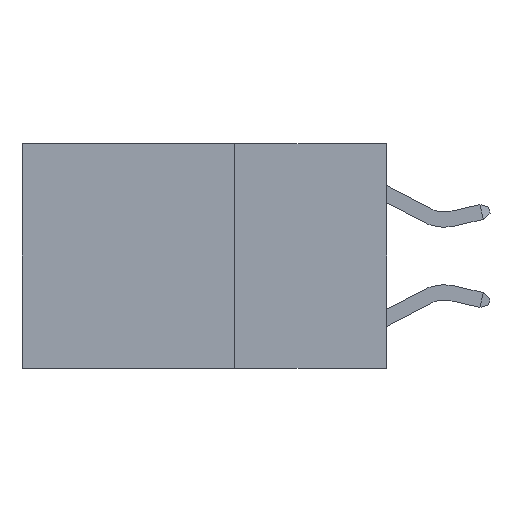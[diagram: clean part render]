
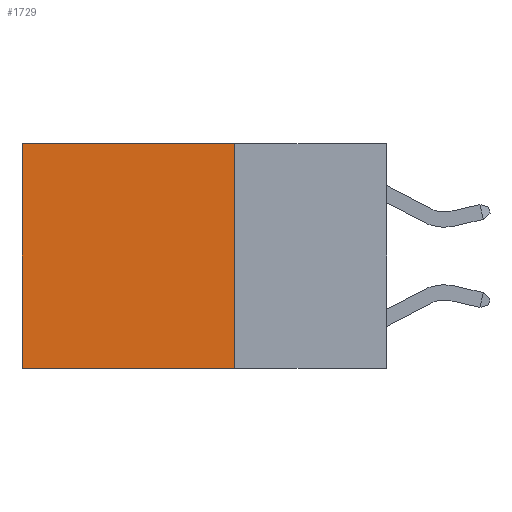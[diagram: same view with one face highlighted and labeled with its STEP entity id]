
A CAD part, left-side view. The second image highlights one B-rep face of the part: STEP entity #1729.
In plain terms, the highlighted planar face has unit normal (-1, 0, 0).
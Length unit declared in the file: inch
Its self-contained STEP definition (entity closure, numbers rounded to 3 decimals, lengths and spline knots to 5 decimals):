
#106 = EDGE_CURVE ( 'NONE', #3373, #7042, #6392, .T. ) ;
#199 = ORIENTED_EDGE ( 'NONE', *, *, #506, .T. ) ;
#506 = EDGE_CURVE ( 'NONE', #5394, #7042, #2859, .T. ) ;
#523 = DIRECTION ( 'NONE',  ( 0., 0., -1. ) ) ;
#618 = ORIENTED_EDGE ( 'NONE', *, *, #106, .F. ) ;
#622 = VECTOR ( 'NONE', #7673, 39.37008 ) ;
#663 = ORIENTED_EDGE ( 'NONE', *, *, #5221, .F. ) ;
#733 = ORIENTED_EDGE ( 'NONE', *, *, #2779, .T. ) ;
#976 = AXIS2_PLACEMENT_3D ( 'NONE', #6938, #6868, #6858 ) ;
#1697 = DIRECTION ( 'NONE',  ( 0., 1., 0. ) ) ;
#1729 = ADVANCED_FACE ( 'NONE', ( #9739 ), #6901, .F. ) ;
#1806 = VERTEX_POINT ( 'NONE', #6404 ) ;
#2435 = DIRECTION ( 'NONE',  ( 0., 1., 0. ) ) ;
#2779 = EDGE_CURVE ( 'NONE', #1806, #5394, #8893, .T. ) ;
#2859 = LINE ( 'NONE', #8277, #622 ) ;
#2938 = VECTOR ( 'NONE', #1697, 39.37008 ) ;
#3373 = VERTEX_POINT ( 'NONE', #6529 ) ;
#5133 = CARTESIAN_POINT ( 'NONE',  ( 0.2625, 0.6, 0. ) ) ;
#5221 = EDGE_CURVE ( 'NONE', #1806, #3373, #5240, .T. ) ;
#5240 = LINE ( 'NONE', #7178, #7122 ) ;
#5394 = VERTEX_POINT ( 'NONE', #5133 ) ;
#6392 = LINE ( 'NONE', #7967, #10524 ) ;
#6404 = CARTESIAN_POINT ( 'NONE',  ( 0.2625, 0.25, 0. ) ) ;
#6529 = CARTESIAN_POINT ( 'NONE',  ( 0.2625, 0.25, -0.37 ) ) ;
#6847 = EDGE_LOOP ( 'NONE', ( #199, #618, #663, #733 ) ) ;
#6858 = DIRECTION ( 'NONE',  ( 0., 0., -1. ) ) ;
#6868 = DIRECTION ( 'NONE',  ( 1., 0., 0. ) ) ;
#6901 = PLANE ( 'NONE',  #976 ) ;
#6938 = CARTESIAN_POINT ( 'NONE',  ( 0.2625, 0.25, 0. ) ) ;
#7042 = VERTEX_POINT ( 'NONE', #8559 ) ;
#7122 = VECTOR ( 'NONE', #523, 39.37008 ) ;
#7178 = CARTESIAN_POINT ( 'NONE',  ( 0.2625, 0.25, 0. ) ) ;
#7490 = CARTESIAN_POINT ( 'NONE',  ( 0.2625, 0.25, 0. ) ) ;
#7673 = DIRECTION ( 'NONE',  ( 0., 0., -1. ) ) ;
#7967 = CARTESIAN_POINT ( 'NONE',  ( 0.2625, 0.25, -0.37 ) ) ;
#8277 = CARTESIAN_POINT ( 'NONE',  ( 0.2625, 0.6, 0. ) ) ;
#8559 = CARTESIAN_POINT ( 'NONE',  ( 0.2625, 0.6, -0.37 ) ) ;
#8893 = LINE ( 'NONE', #7490, #2938 ) ;
#9739 = FACE_OUTER_BOUND ( 'NONE', #6847, .T. ) ;
#10524 = VECTOR ( 'NONE', #2435, 39.37008 ) ;
